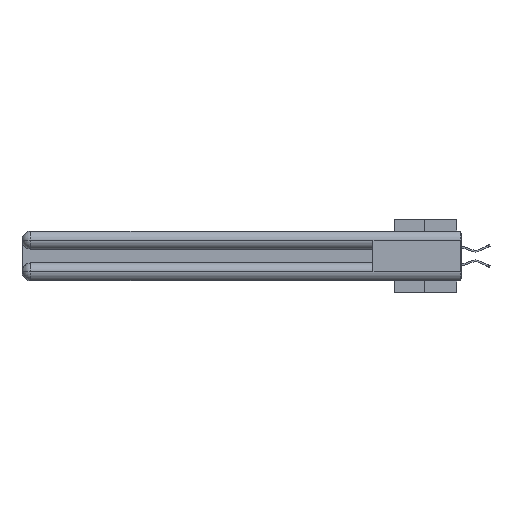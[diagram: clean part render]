
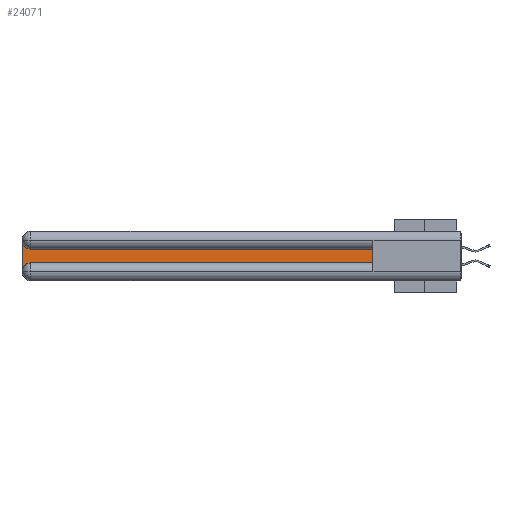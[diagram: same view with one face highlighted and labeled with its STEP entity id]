
A CAD part, left-side view. The second image highlights one B-rep face of the part: STEP entity #24071.
In plain terms, the highlighted planar face has unit normal (-1, 0, 0).
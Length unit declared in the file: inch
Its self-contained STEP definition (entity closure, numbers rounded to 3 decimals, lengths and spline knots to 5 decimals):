
#204 = VECTOR ( 'NONE', #7033, 39.37008 ) ;
#620 = CARTESIAN_POINT ( 'NONE',  ( 0.075, 2.94, -0.2175 ) ) ;
#1784 = LINE ( 'NONE', #17106, #204 ) ;
#3518 = VERTEX_POINT ( 'NONE', #26739 ) ;
#5346 = CARTESIAN_POINT ( 'NONE',  ( 0.075, 2.94, -0.2775 ) ) ;
#5763 = ORIENTED_EDGE ( 'NONE', *, *, #19769, .T. ) ;
#6109 = ORIENTED_EDGE ( 'NONE', *, *, #27665, .T. ) ;
#7033 = DIRECTION ( 'NONE',  ( 0., 0., -1. ) ) ;
#7069 = CARTESIAN_POINT ( 'NONE',  ( 0.075, 0.6, -0.2175 ) ) ;
#7496 = DIRECTION ( 'NONE',  ( 0., 0., -1. ) ) ;
#7825 = DIRECTION ( 'NONE',  ( 0., 0., 1. ) ) ;
#7896 = VERTEX_POINT ( 'NONE', #35288 ) ;
#8277 = EDGE_LOOP ( 'NONE', ( #41837, #17375, #5763, #6109, #41404, #28096 ) ) ;
#8710 = VERTEX_POINT ( 'NONE', #620 ) ;
#8820 = FACE_OUTER_BOUND ( 'NONE', #8277, .T. ) ;
#9084 = EDGE_CURVE ( 'NONE', #8710, #10339, #32350, .T. ) ;
#9639 = EDGE_CURVE ( 'NONE', #10339, #7896, #34857, .T. ) ;
#10339 = VERTEX_POINT ( 'NONE', #29116 ) ;
#10414 = LINE ( 'NONE', #19911, #41467 ) ;
#11908 = DIRECTION ( 'NONE',  ( 0., 0., -1. ) ) ;
#13705 = VERTEX_POINT ( 'NONE', #24306 ) ;
#16538 = DIRECTION ( 'NONE',  ( 1., 0., 0. ) ) ;
#17106 = CARTESIAN_POINT ( 'NONE',  ( 0.075, 3., -0.2175 ) ) ;
#17282 = PLANE ( 'NONE',  #22626 ) ;
#17375 = ORIENTED_EDGE ( 'NONE', *, *, #33353, .T. ) ;
#18135 = EDGE_CURVE ( 'NONE', #7896, #34669, #10414, .T. ) ;
#19769 = EDGE_CURVE ( 'NONE', #13705, #3518, #1784, .T. ) ;
#19780 = CIRCLE ( 'NONE', #33710, 0.06 ) ;
#19911 = CARTESIAN_POINT ( 'NONE',  ( 0.075, 0.6, -0.1225 ) ) ;
#22626 = AXIS2_PLACEMENT_3D ( 'NONE', #31166, #27317, #7496 ) ;
#23272 = VECTOR ( 'NONE', #7825, 39.37008 ) ;
#24071 = ADVANCED_FACE ( 'NONE', ( #8820 ), #17282, .F. ) ;
#24306 = CARTESIAN_POINT ( 'NONE',  ( 0.075, 3., -0.0625 ) ) ;
#25151 = AXIS2_PLACEMENT_3D ( 'NONE', #43428, #16538, #40091 ) ;
#26739 = CARTESIAN_POINT ( 'NONE',  ( 0.075, 3., -0.2775 ) ) ;
#26849 = CARTESIAN_POINT ( 'NONE',  ( 0.075, 0.6, -0.2175 ) ) ;
#27189 = CARTESIAN_POINT ( 'NONE',  ( 0.075, 2.94, -0.1225 ) ) ;
#27317 = DIRECTION ( 'NONE',  ( 1., 0., 0. ) ) ;
#27665 = EDGE_CURVE ( 'NONE', #3518, #8710, #19780, .T. ) ;
#28096 = ORIENTED_EDGE ( 'NONE', *, *, #9639, .T. ) ;
#29116 = CARTESIAN_POINT ( 'NONE',  ( 0.075, 0.6, -0.2175 ) ) ;
#30432 = DIRECTION ( 'NONE',  ( 0., -1., 0. ) ) ;
#31166 = CARTESIAN_POINT ( 'NONE',  ( 0.075, 3., -0.1225 ) ) ;
#32260 = CIRCLE ( 'NONE', #25151, 0.06 ) ;
#32350 = LINE ( 'NONE', #7069, #35483 ) ;
#33353 = EDGE_CURVE ( 'NONE', #34669, #13705, #32260, .T. ) ;
#33710 = AXIS2_PLACEMENT_3D ( 'NONE', #5346, #41760, #11908 ) ;
#34669 = VERTEX_POINT ( 'NONE', #27189 ) ;
#34857 = LINE ( 'NONE', #26849, #23272 ) ;
#35288 = CARTESIAN_POINT ( 'NONE',  ( 0.075, 0.6, -0.1225 ) ) ;
#35483 = VECTOR ( 'NONE', #30432, 39.37008 ) ;
#40091 = DIRECTION ( 'NONE',  ( 0., 0., -1. ) ) ;
#40694 = DIRECTION ( 'NONE',  ( 0., 1., 0. ) ) ;
#41404 = ORIENTED_EDGE ( 'NONE', *, *, #9084, .T. ) ;
#41467 = VECTOR ( 'NONE', #40694, 39.37008 ) ;
#41760 = DIRECTION ( 'NONE',  ( 1., 0., 0. ) ) ;
#41837 = ORIENTED_EDGE ( 'NONE', *, *, #18135, .T. ) ;
#43428 = CARTESIAN_POINT ( 'NONE',  ( 0.075, 2.94, -0.0625 ) ) ;
